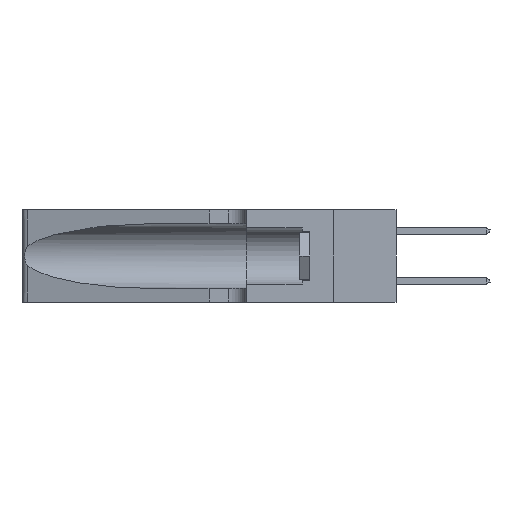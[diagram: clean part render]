
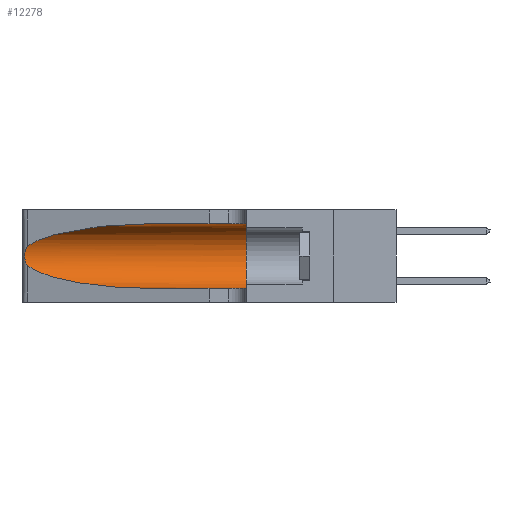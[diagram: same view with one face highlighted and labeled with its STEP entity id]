
A CAD part, left-side view. The second image highlights one B-rep face of the part: STEP entity #12278.
In plain terms, the highlighted cylindrical face has radius 3.308 mm (diameter 6.617 mm), a partial arc.
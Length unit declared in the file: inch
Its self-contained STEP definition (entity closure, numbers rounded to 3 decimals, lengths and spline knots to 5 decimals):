
#112 = DIRECTION ( 'NONE',  ( 0., -1., 0. ) ) ;
#387 = CARTESIAN_POINT ( 'NONE',  ( 0.26075, 1.23896, 0.178 ) ) ;
#1522 = VERTEX_POINT ( 'NONE', #13376 ) ;
#1672 = VERTEX_POINT ( 'NONE', #14807 ) ;
#1697 = CARTESIAN_POINT ( 'NONE',  ( 0.1305, 0.35, 0.185 ) ) ;
#2663 = VECTOR ( 'NONE', #15248, 39.37008 ) ;
#3539 = CARTESIAN_POINT ( 'NONE',  ( 0.2373, 1.15595, 0.08982 ) ) ;
#3757 = CARTESIAN_POINT ( 'NONE',  ( 0.18966, 0.96281, 0.05475 ) ) ;
#3924 = CARTESIAN_POINT ( 'NONE',  ( 0.1305, 1.61858, 0.05475 ) ) ;
#4280 = CARTESIAN_POINT ( 'NONE',  ( 0.25854, 1.2359, 0.20912 ) ) ;
#5018 = CARTESIAN_POINT ( 'NONE',  ( 0.1305, 0.72297, 0.05475 ) ) ;
#5995 = EDGE_LOOP ( 'NONE', ( #23262, #9364, #8069, #15350, #7974, #17704 ) ) ;
#6067 = LINE ( 'NONE', #20641, #2663 ) ;
#6126 = CARTESIAN_POINT ( 'NONE',  ( 0.25639, 1.23184, 0.21858 ) ) ;
#6404 = CARTESIAN_POINT ( 'NONE',  ( 0.2373, 1.15595, 0.28018 ) ) ;
#7207 = EDGE_CURVE ( 'NONE', #22456, #12906, #16621, .T. ) ;
#7353 = AXIS2_PLACEMENT_3D ( 'NONE', #1697, #18067, #16175 ) ;
#7628 = FACE_OUTER_BOUND ( 'NONE', #5995, .T. ) ;
#7974 = ORIENTED_EDGE ( 'NONE', *, *, #14206, .F. ) ;
#8069 = ORIENTED_EDGE ( 'NONE', *, *, #7207, .T. ) ;
#9329 = CYLINDRICAL_SURFACE ( 'NONE', #22329, 0.13025 ) ;
#9364 = ORIENTED_EDGE ( 'NONE', *, *, #14458, .T. ) ;
#9820 = CARTESIAN_POINT ( 'NONE',  ( 0.26018, 1.23835, 0.19895 ) ) ;
#9945 = CARTESIAN_POINT ( 'NONE',  ( 0.18966, 0.96281, 0.31525 ) ) ;
#10113 = EDGE_CURVE ( 'NONE', #1522, #18138, #6067, .T. ) ;
#10725 = VECTOR ( 'NONE', #13033, 39.37008 ) ;
#10732 = CARTESIAN_POINT ( 'NONE',  ( 0.25487, 1.22718, 0.14631 ) ) ;
#11221 = CARTESIAN_POINT ( 'NONE',  ( 0.26075, 1.23896, 0.19203 ) ) ;
#12278 = ADVANCED_FACE ( 'NONE', ( #7628 ), #9329, .F. ) ;
#12392 = CIRCLE ( 'NONE', #7353, 0.13025 ) ;
#12549 = CARTESIAN_POINT ( 'NONE',  ( 0.1305, 0.35, 0.31525 ) ) ;
#12906 = VERTEX_POINT ( 'NONE', #5018 ) ;
#13033 = DIRECTION ( 'NONE',  ( 0., -1., 0. ) ) ;
#13153 =( BOUNDED_CURVE ( )  B_SPLINE_CURVE ( 3, ( #20722, #9945, #6404, #22437 ),
 .UNSPECIFIED., .F., .F. ) 
 B_SPLINE_CURVE_WITH_KNOTS ( ( 4, 4 ),
 ( 1.5708, 2.84003 ),
 .UNSPECIFIED. ) 
 CURVE ( )  GEOMETRIC_REPRESENTATION_ITEM ( )  RATIONAL_B_SPLINE_CURVE ( ( 1., 0.87, 0.87, 1. ) ) 
 REPRESENTATION_ITEM ( '' )  );
#13239 = CARTESIAN_POINT ( 'NONE',  ( 0.25789, 1.23486, 0.15765 ) ) ;
#13376 = CARTESIAN_POINT ( 'NONE',  ( 0.1305, 0.72297, 0.31525 ) ) ;
#13590 = LINE ( 'NONE', #3924, #10725 ) ;
#14206 = EDGE_CURVE ( 'NONE', #18138, #1672, #12392, .T. ) ;
#14458 = EDGE_CURVE ( 'NONE', #14579, #22456, #15638, .T. ) ;
#14579 = VERTEX_POINT ( 'NONE', #20765 ) ;
#14807 = CARTESIAN_POINT ( 'NONE',  ( 0.1305, 0.35, 0.05475 ) ) ;
#14962 = CARTESIAN_POINT ( 'NONE',  ( 0.25856, 1.23593, 0.16098 ) ) ;
#15123 = CARTESIAN_POINT ( 'NONE',  ( 0.25487, 1.22718, 0.14631 ) ) ;
#15207 = CARTESIAN_POINT ( 'NONE',  ( 0.25555, 1.22993, 0.14849 ) ) ;
#15248 = DIRECTION ( 'NONE',  ( 0., -1., 0. ) ) ;
#15350 = ORIENTED_EDGE ( 'NONE', *, *, #16006, .T. ) ;
#15638 = B_SPLINE_CURVE_WITH_KNOTS ( 'NONE', 3,
 ( #18610, #20353, #6126, #20448, #4280, #9820, #11221, #387, #22402, #14962, #13239, #22321, #15207, #15123 ),
 .UNSPECIFIED., .F., .F.,
 ( 4, 2, 2, 2, 2, 2, 4 ),
 ( 0., 0.00027, 0.00053, 0.00107, 0.0016, 0.00187, 0.00214 ),
 .UNSPECIFIED. ) ;
#15819 = CARTESIAN_POINT ( 'NONE',  ( 0.1305, 1.61858, 0.185 ) ) ;
#16006 = EDGE_CURVE ( 'NONE', #12906, #1672, #13590, .T. ) ;
#16175 = DIRECTION ( 'NONE',  ( 0., 0., 1. ) ) ;
#16589 = CARTESIAN_POINT ( 'NONE',  ( 0.25487, 1.22718, 0.14631 ) ) ;
#16621 =( BOUNDED_CURVE ( )  B_SPLINE_CURVE ( 3, ( #10732, #3539, #3757, #18165 ),
 .UNSPECIFIED., .F., .F. ) 
 B_SPLINE_CURVE_WITH_KNOTS ( ( 4, 4 ),
 ( 3.44316, 4.71239 ),
 .UNSPECIFIED. ) 
 CURVE ( )  GEOMETRIC_REPRESENTATION_ITEM ( )  RATIONAL_B_SPLINE_CURVE ( ( 1., 0.87, 0.87, 1. ) ) 
 REPRESENTATION_ITEM ( '' )  );
#17704 = ORIENTED_EDGE ( 'NONE', *, *, #10113, .F. ) ;
#18067 = DIRECTION ( 'NONE',  ( 0., 1., 0. ) ) ;
#18138 = VERTEX_POINT ( 'NONE', #12549 ) ;
#18165 = CARTESIAN_POINT ( 'NONE',  ( 0.1305, 0.72297, 0.05475 ) ) ;
#18610 = CARTESIAN_POINT ( 'NONE',  ( 0.25487, 1.22718, 0.22369 ) ) ;
#18794 = EDGE_CURVE ( 'NONE', #1522, #14579, #13153, .T. ) ;
#19971 = DIRECTION ( 'NONE',  ( 0., 0., -1. ) ) ;
#20353 = CARTESIAN_POINT ( 'NONE',  ( 0.25555, 1.22994, 0.2215 ) ) ;
#20448 = CARTESIAN_POINT ( 'NONE',  ( 0.25787, 1.23484, 0.2124 ) ) ;
#20641 = CARTESIAN_POINT ( 'NONE',  ( 0.1305, 1.61858, 0.31525 ) ) ;
#20722 = CARTESIAN_POINT ( 'NONE',  ( 0.1305, 0.72297, 0.31525 ) ) ;
#20765 = CARTESIAN_POINT ( 'NONE',  ( 0.25487, 1.22718, 0.22369 ) ) ;
#22321 = CARTESIAN_POINT ( 'NONE',  ( 0.25639, 1.23186, 0.15144 ) ) ;
#22329 = AXIS2_PLACEMENT_3D ( 'NONE', #15819, #112, #19971 ) ;
#22402 = CARTESIAN_POINT ( 'NONE',  ( 0.26017, 1.23833, 0.17102 ) ) ;
#22437 = CARTESIAN_POINT ( 'NONE',  ( 0.25487, 1.22718, 0.22369 ) ) ;
#22456 = VERTEX_POINT ( 'NONE', #16589 ) ;
#23262 = ORIENTED_EDGE ( 'NONE', *, *, #18794, .T. ) ;
